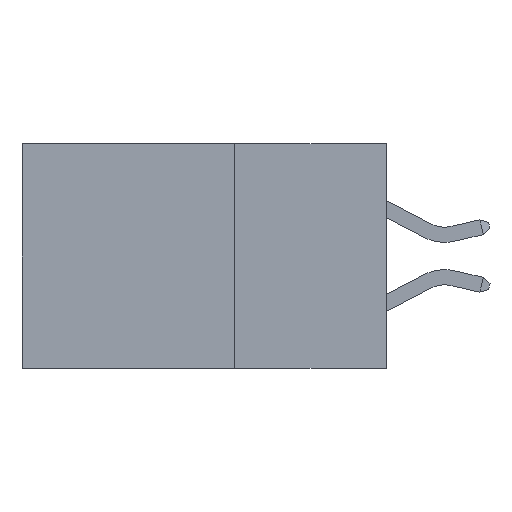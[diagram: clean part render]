
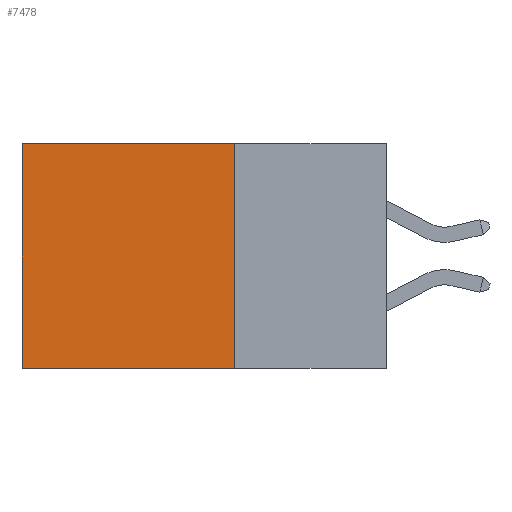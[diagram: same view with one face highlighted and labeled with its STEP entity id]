
A CAD part, left-side view. The second image highlights one B-rep face of the part: STEP entity #7478.
In plain terms, the highlighted planar face has unit normal (-1, 0, 0).
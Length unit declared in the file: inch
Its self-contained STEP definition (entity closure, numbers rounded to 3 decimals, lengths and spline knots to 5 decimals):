
#327 = DIRECTION ( 'NONE',  ( 0., 0., -1. ) ) ;
#1021 = ORIENTED_EDGE ( 'NONE', *, *, #3332, .F. ) ;
#1031 = VECTOR ( 'NONE', #3008, 39.37008 ) ;
#1075 = LINE ( 'NONE', #1382, #5824 ) ;
#1264 = LINE ( 'NONE', #2373, #3524 ) ;
#1382 = CARTESIAN_POINT ( 'NONE',  ( 0.2615, 0.25, 0. ) ) ;
#2076 = ORIENTED_EDGE ( 'NONE', *, *, #10481, .T. ) ;
#2218 = ORIENTED_EDGE ( 'NONE', *, *, #10248, .F. ) ;
#2341 = DIRECTION ( 'NONE',  ( 0., 0., -1. ) ) ;
#2373 = CARTESIAN_POINT ( 'NONE',  ( 0.2615, 0.6, -0.37 ) ) ;
#2550 = EDGE_CURVE ( 'NONE', #9025, #5037, #1264, .T. ) ;
#2947 = CARTESIAN_POINT ( 'NONE',  ( 0.2615, 0.25, -0.37 ) ) ;
#2989 = DIRECTION ( 'NONE',  ( 0., 1., 0. ) ) ;
#3008 = DIRECTION ( 'NONE',  ( 0., 0., -1. ) ) ;
#3041 = CARTESIAN_POINT ( 'NONE',  ( 0.2615, 0.25, -0.37 ) ) ;
#3332 = EDGE_CURVE ( 'NONE', #3348, #5037, #11156, .T. ) ;
#3348 = VERTEX_POINT ( 'NONE', #3041 ) ;
#3524 = VECTOR ( 'NONE', #2341, 39.37008 ) ;
#3811 = VECTOR ( 'NONE', #2989, 39.37008 ) ;
#3893 = LINE ( 'NONE', #7656, #1031 ) ;
#5037 = VERTEX_POINT ( 'NONE', #10482 ) ;
#5171 = DIRECTION ( 'NONE',  ( 0., 1., 0. ) ) ;
#5352 = CARTESIAN_POINT ( 'NONE',  ( 0.2615, 0.25, 0. ) ) ;
#5824 = VECTOR ( 'NONE', #5171, 39.37008 ) ;
#5983 = DIRECTION ( 'NONE',  ( 1., 0., 0. ) ) ;
#6077 = EDGE_LOOP ( 'NONE', ( #10397, #1021, #2218, #2076 ) ) ;
#6282 = AXIS2_PLACEMENT_3D ( 'NONE', #11460, #5983, #327 ) ;
#6675 = VERTEX_POINT ( 'NONE', #5352 ) ;
#6728 = FACE_OUTER_BOUND ( 'NONE', #6077, .T. ) ;
#7478 = ADVANCED_FACE ( 'NONE', ( #6728 ), #10565, .F. ) ;
#7656 = CARTESIAN_POINT ( 'NONE',  ( 0.2615, 0.25, -0.37 ) ) ;
#9025 = VERTEX_POINT ( 'NONE', #9899 ) ;
#9899 = CARTESIAN_POINT ( 'NONE',  ( 0.2615, 0.6, 0. ) ) ;
#10248 = EDGE_CURVE ( 'NONE', #6675, #3348, #3893, .T. ) ;
#10397 = ORIENTED_EDGE ( 'NONE', *, *, #2550, .T. ) ;
#10481 = EDGE_CURVE ( 'NONE', #6675, #9025, #1075, .T. ) ;
#10482 = CARTESIAN_POINT ( 'NONE',  ( 0.2615, 0.6, -0.37 ) ) ;
#10565 = PLANE ( 'NONE',  #6282 ) ;
#11156 = LINE ( 'NONE', #2947, #3811 ) ;
#11460 = CARTESIAN_POINT ( 'NONE',  ( 0.2615, 0.25, -0.37 ) ) ;
